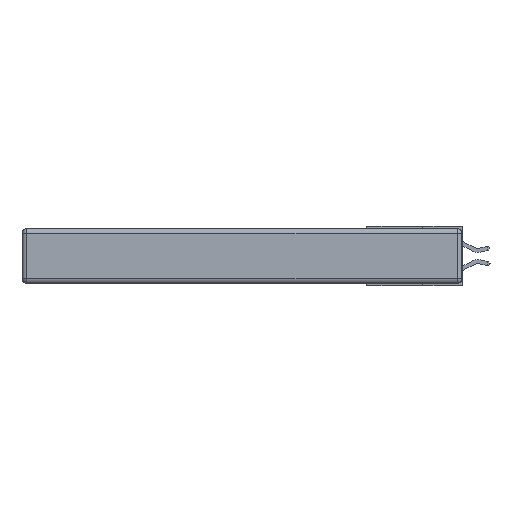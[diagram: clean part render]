
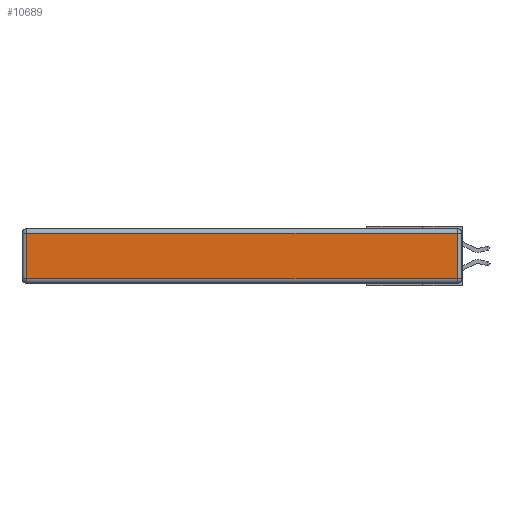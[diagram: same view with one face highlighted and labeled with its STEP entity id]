
A CAD part, left-side view. The second image highlights one B-rep face of the part: STEP entity #10689.
In plain terms, the highlighted planar face has unit normal (-1, 0, 0).
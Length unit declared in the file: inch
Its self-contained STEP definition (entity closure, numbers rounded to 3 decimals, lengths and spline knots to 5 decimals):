
#688 = ORIENTED_EDGE ( 'NONE', *, *, #13167, .T. ) ;
#797 = ORIENTED_EDGE ( 'NONE', *, *, #8692, .T. ) ;
#1933 = VECTOR ( 'NONE', #9229, 39.37008 ) ;
#2368 = VERTEX_POINT ( 'NONE', #3069 ) ;
#2551 = VECTOR ( 'NONE', #18278, 39.37008 ) ;
#2993 = CARTESIAN_POINT ( 'NONE',  ( 0., 0., -0.343 ) ) ;
#3069 = CARTESIAN_POINT ( 'NONE',  ( 0., 2.72, -0.03 ) ) ;
#3534 = CARTESIAN_POINT ( 'NONE',  ( 0., 2.75, -0.03 ) ) ;
#3608 = ORIENTED_EDGE ( 'NONE', *, *, #19300, .T. ) ;
#3895 = VECTOR ( 'NONE', #15811, 39.37008 ) ;
#4002 = VERTEX_POINT ( 'NONE', #5084 ) ;
#5084 = CARTESIAN_POINT ( 'NONE',  ( 0., 0.03, -0.03 ) ) ;
#5266 = CARTESIAN_POINT ( 'NONE',  ( 0., 0.03, -0.313 ) ) ;
#5747 = CARTESIAN_POINT ( 'NONE',  ( 0., 2.72, -0.343 ) ) ;
#6086 = PLANE ( 'NONE',  #12284 ) ;
#7152 = CARTESIAN_POINT ( 'NONE',  ( 0., 2.72, -0.313 ) ) ;
#7511 = DIRECTION ( 'NONE',  ( 0., 0., 1. ) ) ;
#7562 = CARTESIAN_POINT ( 'NONE',  ( 0., 0.03, -0.343 ) ) ;
#8251 = DIRECTION ( 'NONE',  ( 0., -1., 0. ) ) ;
#8692 = EDGE_CURVE ( 'NONE', #18208, #4002, #14986, .T. ) ;
#9229 = DIRECTION ( 'NONE',  ( 0., 0., 1. ) ) ;
#10540 = LINE ( 'NONE', #14392, #14418 ) ;
#10541 = FACE_OUTER_BOUND ( 'NONE', #11547, .T. ) ;
#10689 = ADVANCED_FACE ( 'NONE', ( #10541 ), #6086, .T. ) ;
#11547 = EDGE_LOOP ( 'NONE', ( #3608, #797, #13968, #688 ) ) ;
#12284 = AXIS2_PLACEMENT_3D ( 'NONE', #2993, #16909, #7511 ) ;
#13167 = EDGE_CURVE ( 'NONE', #2368, #17337, #15127, .T. ) ;
#13968 = ORIENTED_EDGE ( 'NONE', *, *, #16797, .T. ) ;
#14392 = CARTESIAN_POINT ( 'NONE',  ( 0., 0., -0.313 ) ) ;
#14418 = VECTOR ( 'NONE', #8251, 39.37008 ) ;
#14986 = LINE ( 'NONE', #7562, #1933 ) ;
#15127 = LINE ( 'NONE', #5747, #2551 ) ;
#15811 = DIRECTION ( 'NONE',  ( 0., 1., 0. ) ) ;
#16797 = EDGE_CURVE ( 'NONE', #4002, #2368, #19168, .T. ) ;
#16909 = DIRECTION ( 'NONE',  ( -1., 0., 0. ) ) ;
#17337 = VERTEX_POINT ( 'NONE', #7152 ) ;
#18208 = VERTEX_POINT ( 'NONE', #5266 ) ;
#18278 = DIRECTION ( 'NONE',  ( 0., 0., -1. ) ) ;
#19168 = LINE ( 'NONE', #3534, #3895 ) ;
#19300 = EDGE_CURVE ( 'NONE', #17337, #18208, #10540, .T. ) ;
